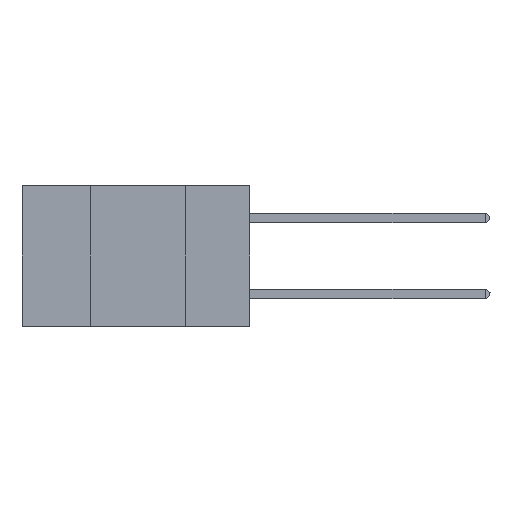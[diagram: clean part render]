
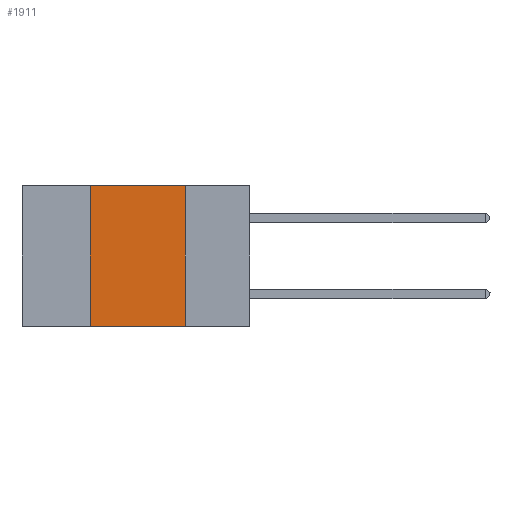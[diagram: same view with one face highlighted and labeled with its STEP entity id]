
A CAD part, left-side view. The second image highlights one B-rep face of the part: STEP entity #1911.
In plain terms, the highlighted planar face has unit normal (-1, 0, 0).
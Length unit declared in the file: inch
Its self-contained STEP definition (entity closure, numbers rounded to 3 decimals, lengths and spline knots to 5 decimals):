
#196 = CARTESIAN_POINT ( 'NONE',  ( 0., 0.42, -0.37 ) ) ;
#337 = ORIENTED_EDGE ( 'NONE', *, *, #8012, .F. ) ;
#631 = DIRECTION ( 'NONE',  ( 0., -1., 0. ) ) ;
#685 = VECTOR ( 'NONE', #2116, 39.37008 ) ;
#1888 = LINE ( 'NONE', #30135, #6237 ) ;
#1911 = ADVANCED_FACE ( 'NONE', ( #26498 ), #20440, .F. ) ;
#2116 = DIRECTION ( 'NONE',  ( 0., -1., 0. ) ) ;
#2825 = CARTESIAN_POINT ( 'NONE',  ( 0., 0.6, 0. ) ) ;
#4384 = AXIS2_PLACEMENT_3D ( 'NONE', #2825, #8692, #34656 ) ;
#5459 = CARTESIAN_POINT ( 'NONE',  ( 0., 0.42, 0. ) ) ;
#6237 = VECTOR ( 'NONE', #10411, 39.37008 ) ;
#6308 = CARTESIAN_POINT ( 'NONE',  ( 0., 0.6, -0.37 ) ) ;
#6723 = EDGE_CURVE ( 'NONE', #33776, #35387, #1888, .T. ) ;
#6910 = VECTOR ( 'NONE', #631, 39.37008 ) ;
#8012 = EDGE_CURVE ( 'NONE', #15612, #16419, #8113, .T. ) ;
#8113 = LINE ( 'NONE', #36790, #23783 ) ;
#8692 = DIRECTION ( 'NONE',  ( 1., 0., 0. ) ) ;
#9653 = EDGE_CURVE ( 'NONE', #33776, #16419, #32641, .T. ) ;
#10411 = DIRECTION ( 'NONE',  ( 0., 0., 1. ) ) ;
#15449 = CARTESIAN_POINT ( 'NONE',  ( 0., 0.6, 0. ) ) ;
#15612 = VERTEX_POINT ( 'NONE', #23616 ) ;
#16419 = VERTEX_POINT ( 'NONE', #37256 ) ;
#16516 = DIRECTION ( 'NONE',  ( 0., 0., -1. ) ) ;
#16771 = ORIENTED_EDGE ( 'NONE', *, *, #6723, .F. ) ;
#17144 = EDGE_LOOP ( 'NONE', ( #337, #23941, #16771, #23590 ) ) ;
#20440 = PLANE ( 'NONE',  #4384 ) ;
#23590 = ORIENTED_EDGE ( 'NONE', *, *, #9653, .T. ) ;
#23616 = CARTESIAN_POINT ( 'NONE',  ( 0., 0.17, 0. ) ) ;
#23783 = VECTOR ( 'NONE', #16516, 39.37008 ) ;
#23941 = ORIENTED_EDGE ( 'NONE', *, *, #36110, .F. ) ;
#26498 = FACE_OUTER_BOUND ( 'NONE', #17144, .T. ) ;
#30135 = CARTESIAN_POINT ( 'NONE',  ( 0., 0.42, 0. ) ) ;
#31111 = LINE ( 'NONE', #15449, #685 ) ;
#32641 = LINE ( 'NONE', #6308, #6910 ) ;
#33776 = VERTEX_POINT ( 'NONE', #196 ) ;
#34656 = DIRECTION ( 'NONE',  ( 0., 0., -1. ) ) ;
#35387 = VERTEX_POINT ( 'NONE', #5459 ) ;
#36110 = EDGE_CURVE ( 'NONE', #35387, #15612, #31111, .T. ) ;
#36790 = CARTESIAN_POINT ( 'NONE',  ( 0., 0.17, 0. ) ) ;
#37256 = CARTESIAN_POINT ( 'NONE',  ( 0., 0.17, -0.37 ) ) ;
